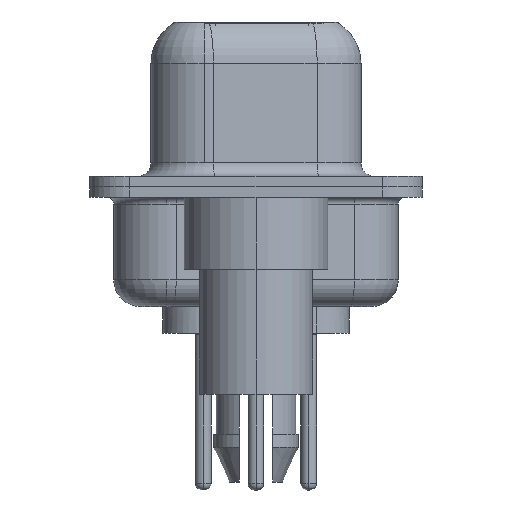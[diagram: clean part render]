
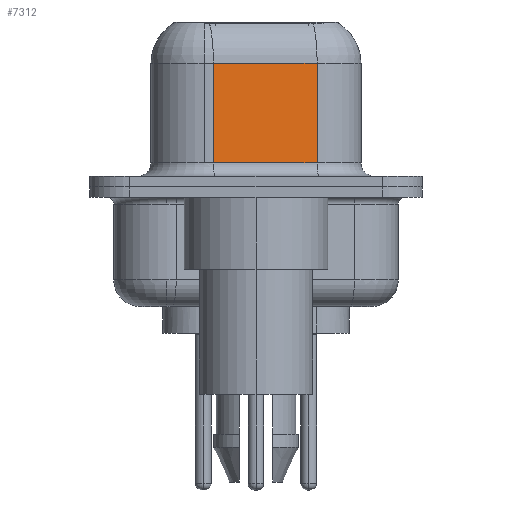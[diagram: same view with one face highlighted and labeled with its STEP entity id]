
A CAD part, left-side view. The second image highlights one B-rep face of the part: STEP entity #7312.
In plain terms, the highlighted planar face has unit normal (-0.985, -0.174, 0).
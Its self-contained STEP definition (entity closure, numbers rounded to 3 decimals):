
#1253 = VECTOR ( 'NONE', #18751, 1000. ) ;
#1674 = CARTESIAN_POINT ( 'NONE',  ( 4.38, 1.603, 0.9 ) ) ;
#2304 = CARTESIAN_POINT ( 'NONE',  ( 5.068, -2.297, 0.9 ) ) ;
#2334 = CARTESIAN_POINT ( 'NONE',  ( 5.068, -2.297, 4.65 ) ) ;
#2424 = VECTOR ( 'NONE', #17966, 1000. ) ;
#2656 = ORIENTED_EDGE ( 'NONE', *, *, #15543, .T. ) ;
#2683 = CARTESIAN_POINT ( 'NONE',  ( 5.068, -2.297, 0.9 ) ) ;
#2783 = DIRECTION ( 'NONE',  ( 0.174, -0.985, 0. ) ) ;
#3091 = VERTEX_POINT ( 'NONE', #18870 ) ;
#3577 = EDGE_CURVE ( 'NONE', #13137, #3091, #18165, .T. ) ;
#7312 = ADVANCED_FACE ( 'NONE', ( #19100 ), #17381, .F. ) ;
#7743 = EDGE_CURVE ( 'NONE', #13137, #13601, #7758, .T. ) ;
#7758 = LINE ( 'NONE', #13957, #1253 ) ;
#7826 = VECTOR ( 'NONE', #14849, 1000. ) ;
#8823 = EDGE_LOOP ( 'NONE', ( #16726, #15403, #18931, #2656 ) ) ;
#9976 = CARTESIAN_POINT ( 'NONE',  ( 4.38, 1.603, 6.4 ) ) ;
#11363 = DIRECTION ( 'NONE',  ( -0.174, 0.985, 0. ) ) ;
#13137 = VERTEX_POINT ( 'NONE', #18891 ) ;
#13601 = VERTEX_POINT ( 'NONE', #2304 ) ;
#13957 = CARTESIAN_POINT ( 'NONE',  ( 5.068, -2.297, 6.4 ) ) ;
#14042 = EDGE_CURVE ( 'NONE', #3091, #15185, #16393, .T. ) ;
#14849 = DIRECTION ( 'NONE',  ( 0., 0., -1. ) ) ;
#15185 = VERTEX_POINT ( 'NONE', #1674 ) ;
#15403 = ORIENTED_EDGE ( 'NONE', *, *, #3577, .T. ) ;
#15543 = EDGE_CURVE ( 'NONE', #15185, #13601, #19750, .T. ) ;
#16114 = AXIS2_PLACEMENT_3D ( 'NONE', #17172, #17272, #11363 ) ;
#16393 = LINE ( 'NONE', #9976, #7826 ) ;
#16726 = ORIENTED_EDGE ( 'NONE', *, *, #7743, .F. ) ;
#17172 = CARTESIAN_POINT ( 'NONE',  ( 5.068, -2.297, 6.4 ) ) ;
#17272 = DIRECTION ( 'NONE',  ( 0.985, 0.174, 0. ) ) ;
#17309 = VECTOR ( 'NONE', #2783, 1000. ) ;
#17381 = PLANE ( 'NONE',  #16114 ) ;
#17966 = DIRECTION ( 'NONE',  ( -0.174, 0.985, 0. ) ) ;
#18165 = LINE ( 'NONE', #2334, #2424 ) ;
#18751 = DIRECTION ( 'NONE',  ( 0., 0., -1. ) ) ;
#18870 = CARTESIAN_POINT ( 'NONE',  ( 4.38, 1.603, 4.65 ) ) ;
#18891 = CARTESIAN_POINT ( 'NONE',  ( 5.068, -2.297, 4.65 ) ) ;
#18931 = ORIENTED_EDGE ( 'NONE', *, *, #14042, .T. ) ;
#19100 = FACE_OUTER_BOUND ( 'NONE', #8823, .T. ) ;
#19750 = LINE ( 'NONE', #2683, #17309 ) ;
